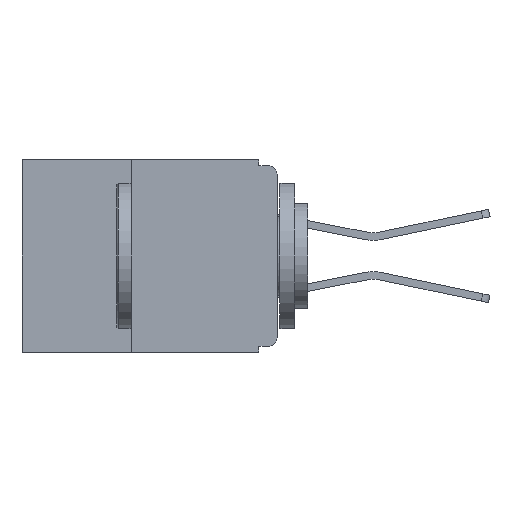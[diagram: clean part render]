
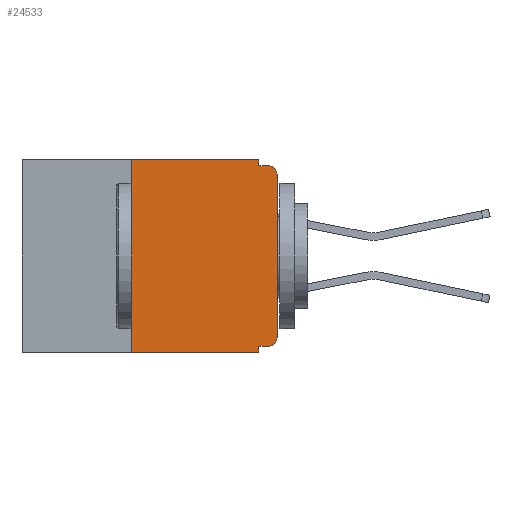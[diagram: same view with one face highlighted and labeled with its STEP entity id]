
A CAD part, left-side view. The second image highlights one B-rep face of the part: STEP entity #24533.
In plain terms, the highlighted planar face has unit normal (-1, 0, 0).
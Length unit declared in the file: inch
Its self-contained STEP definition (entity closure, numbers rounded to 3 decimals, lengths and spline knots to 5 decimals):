
#850 = LINE ( 'NONE', #10524, #7218 ) ;
#1360 = CARTESIAN_POINT ( 'NONE',  ( 0., 0.031, -0.33 ) ) ;
#1375 = CARTESIAN_POINT ( 'NONE',  ( 0., 0.437, -0.33 ) ) ;
#2320 = DIRECTION ( 'NONE',  ( -1., 0., 0. ) ) ;
#2474 = EDGE_CURVE ( 'NONE', #26540, #7212, #850, .T. ) ;
#2514 = CARTESIAN_POINT ( 'NONE',  ( 0., 0.25, 0. ) ) ;
#4514 = CARTESIAN_POINT ( 'NONE',  ( 0., 0.031, 0. ) ) ;
#4566 = EDGE_CURVE ( 'NONE', #17277, #24713, #17027, .T. ) ;
#4915 = ORIENTED_EDGE ( 'NONE', *, *, #23038, .T. ) ;
#4920 = DIRECTION ( 'NONE',  ( 0., 0., 1. ) ) ;
#6829 = VECTOR ( 'NONE', #4920, 39.37008 ) ;
#6916 = VERTEX_POINT ( 'NONE', #16180 ) ;
#6929 = EDGE_CURVE ( 'NONE', #24713, #26540, #9197, .T. ) ;
#7141 = EDGE_CURVE ( 'NONE', #11535, #8587, #10292, .T. ) ;
#7212 = VERTEX_POINT ( 'NONE', #11536 ) ;
#7218 = VECTOR ( 'NONE', #17290, 39.37008 ) ;
#8587 = VERTEX_POINT ( 'NONE', #25448 ) ;
#9197 = LINE ( 'NONE', #15590, #20987 ) ;
#9280 = CIRCLE ( 'NONE', #28263, 0.015 ) ;
#9290 = AXIS2_PLACEMENT_3D ( 'NONE', #12205, #12174, #12108 ) ;
#9764 = CARTESIAN_POINT ( 'NONE',  ( 0., 0., 0. ) ) ;
#10191 = ORIENTED_EDGE ( 'NONE', *, *, #12383, .F. ) ;
#10292 = CIRCLE ( 'NONE', #9290, 0.015 ) ;
#10318 = LINE ( 'NONE', #29467, #13556 ) ;
#10524 = CARTESIAN_POINT ( 'NONE',  ( 0., 0., -0.01 ) ) ;
#10829 = LINE ( 'NONE', #29195, #28008 ) ;
#10830 = VECTOR ( 'NONE', #14111, 39.37008 ) ;
#10920 = VECTOR ( 'NONE', #13911, 39.37008 ) ;
#11535 = VERTEX_POINT ( 'NONE', #19680 ) ;
#11536 = CARTESIAN_POINT ( 'NONE',  ( 0., 0.015, -0.01 ) ) ;
#12012 = ORIENTED_EDGE ( 'NONE', *, *, #2474, .F. ) ;
#12108 = DIRECTION ( 'NONE',  ( 0., 0., -1. ) ) ;
#12174 = DIRECTION ( 'NONE',  ( -1., 0., 0. ) ) ;
#12205 = CARTESIAN_POINT ( 'NONE',  ( 0., 0.015, -0.305 ) ) ;
#12383 = EDGE_CURVE ( 'NONE', #13364, #17615, #10318, .T. ) ;
#13364 = VERTEX_POINT ( 'NONE', #28496 ) ;
#13556 = VECTOR ( 'NONE', #24933, 39.37008 ) ;
#13911 = DIRECTION ( 'NONE',  ( 0., 0., 1. ) ) ;
#14111 = DIRECTION ( 'NONE',  ( 0., -1., 0. ) ) ;
#14811 = CARTESIAN_POINT ( 'NONE',  ( 0., 0.437, 0. ) ) ;
#14926 = ORIENTED_EDGE ( 'NONE', *, *, #4566, .F. ) ;
#15417 = DIRECTION ( 'NONE',  ( 0., 0., -1. ) ) ;
#15590 = CARTESIAN_POINT ( 'NONE',  ( 0., 0.031, 0. ) ) ;
#15713 = DIRECTION ( 'NONE',  ( 0., 0., -1. ) ) ;
#15903 = CARTESIAN_POINT ( 'NONE',  ( 0., 0.25, -0.33 ) ) ;
#16180 = CARTESIAN_POINT ( 'NONE',  ( 0., 0., -0.025 ) ) ;
#16488 = CARTESIAN_POINT ( 'NONE',  ( 0., 0.015, -0.025 ) ) ;
#17027 = LINE ( 'NONE', #14811, #10830 ) ;
#17119 = LINE ( 'NONE', #30263, #10920 ) ;
#17277 = VERTEX_POINT ( 'NONE', #2514 ) ;
#17290 = DIRECTION ( 'NONE',  ( 0., -1., 0. ) ) ;
#17560 = DIRECTION ( 'NONE',  ( 0., 1., 0. ) ) ;
#17615 = VERTEX_POINT ( 'NONE', #1360 ) ;
#17989 = PLANE ( 'NONE',  #24363 ) ;
#18903 = DIRECTION ( 'NONE',  ( 0., 0., -1. ) ) ;
#19392 = LINE ( 'NONE', #9764, #6829 ) ;
#19629 = EDGE_CURVE ( 'NONE', #11535, #13364, #10829, .T. ) ;
#19669 = FACE_OUTER_BOUND ( 'NONE', #24983, .T. ) ;
#19680 = CARTESIAN_POINT ( 'NONE',  ( 0., 0.015, -0.32 ) ) ;
#20364 = DIRECTION ( 'NONE',  ( 0., -1., 0. ) ) ;
#20987 = VECTOR ( 'NONE', #15417, 39.37008 ) ;
#21963 = ORIENTED_EDGE ( 'NONE', *, *, #22381, .F. ) ;
#22381 = EDGE_CURVE ( 'NONE', #25622, #17277, #17119, .T. ) ;
#23038 = EDGE_CURVE ( 'NONE', #8587, #6916, #19392, .T. ) ;
#23781 = ORIENTED_EDGE ( 'NONE', *, *, #25789, .T. ) ;
#24150 = ORIENTED_EDGE ( 'NONE', *, *, #7141, .T. ) ;
#24363 = AXIS2_PLACEMENT_3D ( 'NONE', #25054, #29691, #15713 ) ;
#24533 = ADVANCED_FACE ( 'NONE', ( #19669 ), #17989, .F. ) ;
#24713 = VERTEX_POINT ( 'NONE', #4514 ) ;
#24933 = DIRECTION ( 'NONE',  ( 0., 0., -1. ) ) ;
#24983 = EDGE_LOOP ( 'NONE', ( #4915, #23781, #12012, #25209, #14926, #21963, #28118, #10191, #29558, #24150 ) ) ;
#25054 = CARTESIAN_POINT ( 'NONE',  ( 0., 0.437, 0. ) ) ;
#25114 = EDGE_CURVE ( 'NONE', #25622, #17615, #29058, .T. ) ;
#25209 = ORIENTED_EDGE ( 'NONE', *, *, #6929, .F. ) ;
#25448 = CARTESIAN_POINT ( 'NONE',  ( 0., 0., -0.305 ) ) ;
#25622 = VERTEX_POINT ( 'NONE', #15903 ) ;
#25789 = EDGE_CURVE ( 'NONE', #6916, #7212, #9280, .T. ) ;
#26540 = VERTEX_POINT ( 'NONE', #28822 ) ;
#27611 = VECTOR ( 'NONE', #20364, 39.37008 ) ;
#28008 = VECTOR ( 'NONE', #17560, 39.37008 ) ;
#28118 = ORIENTED_EDGE ( 'NONE', *, *, #25114, .T. ) ;
#28263 = AXIS2_PLACEMENT_3D ( 'NONE', #16488, #2320, #18903 ) ;
#28496 = CARTESIAN_POINT ( 'NONE',  ( 0., 0.031, -0.32 ) ) ;
#28822 = CARTESIAN_POINT ( 'NONE',  ( 0., 0.031, -0.01 ) ) ;
#29058 = LINE ( 'NONE', #1375, #27611 ) ;
#29195 = CARTESIAN_POINT ( 'NONE',  ( 0., 0., -0.32 ) ) ;
#29467 = CARTESIAN_POINT ( 'NONE',  ( 0., 0.031, -0.33 ) ) ;
#29558 = ORIENTED_EDGE ( 'NONE', *, *, #19629, .F. ) ;
#29691 = DIRECTION ( 'NONE',  ( 1., 0., 0. ) ) ;
#30263 = CARTESIAN_POINT ( 'NONE',  ( 0., 0.25, -0.33 ) ) ;
